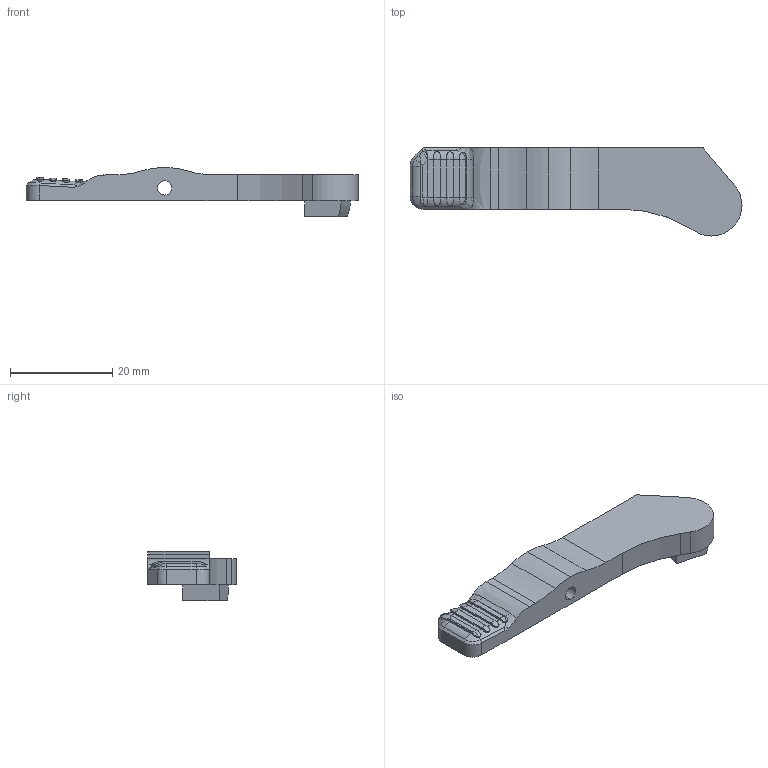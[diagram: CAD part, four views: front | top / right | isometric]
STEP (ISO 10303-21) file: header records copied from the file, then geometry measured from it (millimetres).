
FILE_DESCRIPTION (( 'STEP AP203' ), '1' );
FILE_NAME ('AR-9 Mag Catch V1.0.STEP', '2021-12-24T01:33:12', ( '' ), ( '' ), 'SwSTEP 2.0', 'SolidWorks 2021', '' );
FILE_SCHEMA (( 'CONFIG_CONTROL_DESIGN' ));
Length unit declared in the file: inch
Products named in the file (1): AR-9 Mag Catch V1.0
Bounding box: 64.79 x 17.19 x 9.56 mm (x, y, z)
Volume: 4017.2 mm3; surface area: 2541.4 mm2
Topology: 1 solids, 1 shells, 173 faces, 427 edges, 259 vertices
Faces by surface type: bspline 100, cylinder 35, plane 31, torus 7
Entity records: 12134 total; most frequent: CARTESIAN_POINT 8844, ORIENTED_EDGE 852, EDGE_CURVE 426, DIRECTION 342, B_SPLINE_CURVE_WITH_KNOTS 263, VERTEX_POINT 259, EDGE_LOOP 179, FACE_OUTER_BOUND 173
